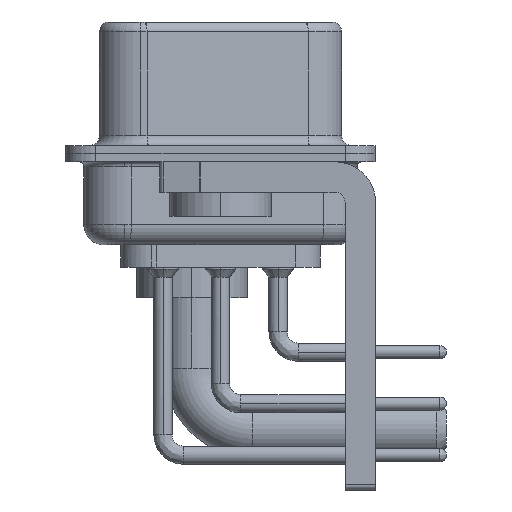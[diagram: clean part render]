
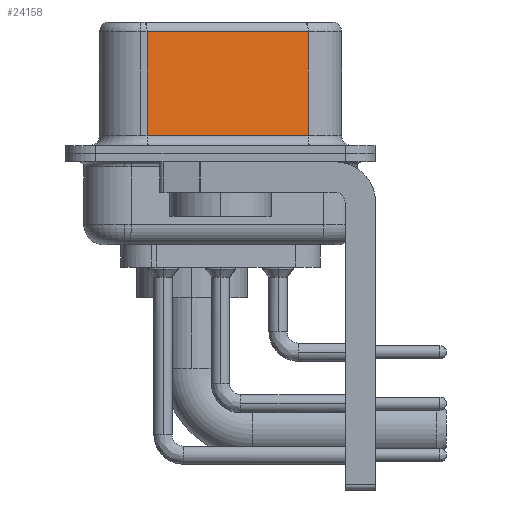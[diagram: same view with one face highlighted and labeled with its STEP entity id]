
A CAD part, left-side view. The second image highlights one B-rep face of the part: STEP entity #24158.
In plain terms, the highlighted planar face has unit normal (-0.985, -0.174, 0).
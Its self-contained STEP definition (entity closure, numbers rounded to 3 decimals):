
#173 = FACE_OUTER_BOUND ( 'NONE', #2519, .T. ) ;
#314 = LINE ( 'NONE', #25182, #3721 ) ;
#603 = DIRECTION ( 'NONE',  ( 0.174, -0.985, 0. ) ) ;
#1206 = AXIS2_PLACEMENT_3D ( 'NONE', #34605, #2605, #10894 ) ;
#2519 = EDGE_LOOP ( 'NONE', ( #12048, #23376, #25440, #33374 ) ) ;
#2527 = VECTOR ( 'NONE', #31821, 1000. ) ;
#2605 = DIRECTION ( 'NONE',  ( 0.985, 0.174, 0. ) ) ;
#2871 = EDGE_CURVE ( 'NONE', #30132, #17202, #5300, .T. ) ;
#3721 = VECTOR ( 'NONE', #16734, 1000. ) ;
#5300 = LINE ( 'NONE', #19946, #35129 ) ;
#8697 = CARTESIAN_POINT ( 'NONE',  ( 5.132, -4.322, 6.52 ) ) ;
#10894 = DIRECTION ( 'NONE',  ( -0.174, 0.985, 0. ) ) ;
#11640 = PLANE ( 'NONE',  #1206 ) ;
#12048 = ORIENTED_EDGE ( 'NONE', *, *, #29441, .F. ) ;
#12064 = CARTESIAN_POINT ( 'NONE',  ( 5.132, -4.322, 0.9 ) ) ;
#14414 = CARTESIAN_POINT ( 'NONE',  ( 5.132, -4.322, 6.02 ) ) ;
#14528 = LINE ( 'NONE', #8697, #2527 ) ;
#15708 = VERTEX_POINT ( 'NONE', #36257 ) ;
#16734 = DIRECTION ( 'NONE',  ( 0., 0., -1. ) ) ;
#17202 = VERTEX_POINT ( 'NONE', #17942 ) ;
#17329 = LINE ( 'NONE', #12064, #35145 ) ;
#17942 = CARTESIAN_POINT ( 'NONE',  ( 3.73, 3.628, 6.02 ) ) ;
#19946 = CARTESIAN_POINT ( 'NONE',  ( 5.132, -4.322, 6.02 ) ) ;
#22044 = DIRECTION ( 'NONE',  ( -0.174, 0.985, 0. ) ) ;
#23376 = ORIENTED_EDGE ( 'NONE', *, *, #2871, .T. ) ;
#24158 = ADVANCED_FACE ( 'NONE', ( #173 ), #11640, .F. ) ;
#25182 = CARTESIAN_POINT ( 'NONE',  ( 3.73, 3.628, 6.52 ) ) ;
#25440 = ORIENTED_EDGE ( 'NONE', *, *, #27294, .T. ) ;
#27294 = EDGE_CURVE ( 'NONE', #17202, #15708, #314, .T. ) ;
#29441 = EDGE_CURVE ( 'NONE', #30132, #36650, #14528, .T. ) ;
#30132 = VERTEX_POINT ( 'NONE', #14414 ) ;
#31371 = CARTESIAN_POINT ( 'NONE',  ( 5.132, -4.322, 0.9 ) ) ;
#31821 = DIRECTION ( 'NONE',  ( 0., 0., -1. ) ) ;
#33353 = EDGE_CURVE ( 'NONE', #15708, #36650, #17329, .T. ) ;
#33374 = ORIENTED_EDGE ( 'NONE', *, *, #33353, .T. ) ;
#34605 = CARTESIAN_POINT ( 'NONE',  ( 5.132, -4.322, 6.52 ) ) ;
#35129 = VECTOR ( 'NONE', #22044, 1000. ) ;
#35145 = VECTOR ( 'NONE', #603, 1000. ) ;
#36257 = CARTESIAN_POINT ( 'NONE',  ( 3.73, 3.628, 0.9 ) ) ;
#36650 = VERTEX_POINT ( 'NONE', #31371 ) ;
